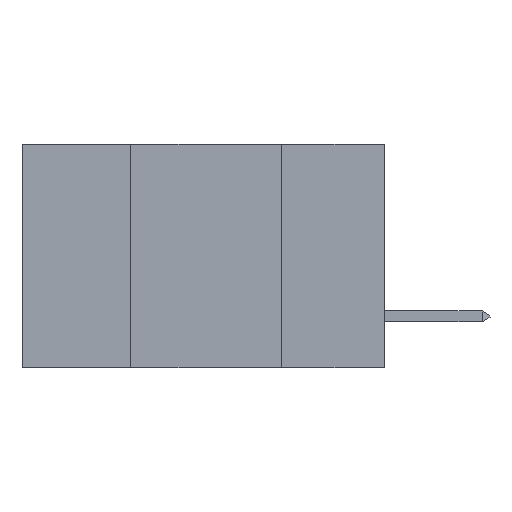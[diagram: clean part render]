
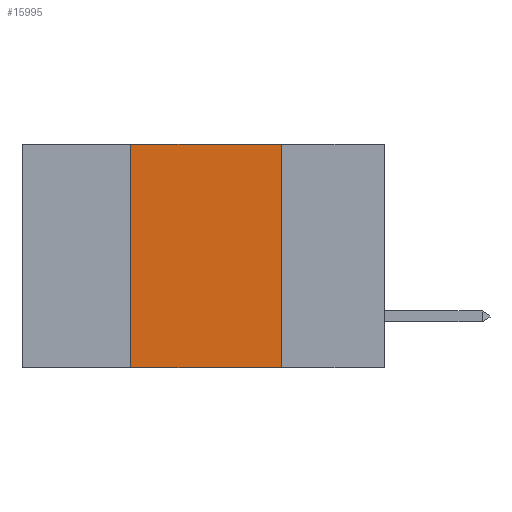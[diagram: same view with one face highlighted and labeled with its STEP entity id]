
A CAD part, left-side view. The second image highlights one B-rep face of the part: STEP entity #15995.
In plain terms, the highlighted planar face has unit normal (-1, 0, 0).
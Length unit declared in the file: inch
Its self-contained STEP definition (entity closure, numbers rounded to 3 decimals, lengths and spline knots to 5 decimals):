
#374 = EDGE_CURVE ( 'NONE', #13476, #15386, #3589, .T. ) ;
#1510 = CARTESIAN_POINT ( 'NONE',  ( 0., 0.42, -0.37 ) ) ;
#1744 = DIRECTION ( 'NONE',  ( 0., 0., 1. ) ) ;
#2388 = CARTESIAN_POINT ( 'NONE',  ( 0., 0.42, 0. ) ) ;
#2417 = EDGE_CURVE ( 'NONE', #13632, #15386, #13837, .T. ) ;
#2480 = DIRECTION ( 'NONE',  ( 0., -1., 0. ) ) ;
#3125 = VECTOR ( 'NONE', #2480, 39.37008 ) ;
#3589 = LINE ( 'NONE', #6136, #9292 ) ;
#3931 = CARTESIAN_POINT ( 'NONE',  ( 0., 0.6, 0. ) ) ;
#4759 = ORIENTED_EDGE ( 'NONE', *, *, #2417, .T. ) ;
#5179 = VECTOR ( 'NONE', #1744, 39.37008 ) ;
#5359 = ORIENTED_EDGE ( 'NONE', *, *, #374, .F. ) ;
#6024 = DIRECTION ( 'NONE',  ( 0., 0., -1. ) ) ;
#6128 = CARTESIAN_POINT ( 'NONE',  ( 0., 0.42, 0. ) ) ;
#6136 = CARTESIAN_POINT ( 'NONE',  ( 0., 0.17, 0. ) ) ;
#6312 = VERTEX_POINT ( 'NONE', #2388 ) ;
#6622 = DIRECTION ( 'NONE',  ( 0., -1., 0. ) ) ;
#7941 = LINE ( 'NONE', #13098, #18543 ) ;
#8242 = DIRECTION ( 'NONE',  ( 1., 0., 0. ) ) ;
#9292 = VECTOR ( 'NONE', #6024, 39.37008 ) ;
#10868 = LINE ( 'NONE', #6128, #5179 ) ;
#12105 = EDGE_CURVE ( 'NONE', #6312, #13476, #7941, .T. ) ;
#13098 = CARTESIAN_POINT ( 'NONE',  ( 0., 0.6, 0. ) ) ;
#13476 = VERTEX_POINT ( 'NONE', #17970 ) ;
#13632 = VERTEX_POINT ( 'NONE', #1510 ) ;
#13837 = LINE ( 'NONE', #17589, #3125 ) ;
#14036 = ORIENTED_EDGE ( 'NONE', *, *, #12105, .F. ) ;
#14387 = CARTESIAN_POINT ( 'NONE',  ( 0., 0.17, -0.37 ) ) ;
#15386 = VERTEX_POINT ( 'NONE', #14387 ) ;
#15995 = ADVANCED_FACE ( 'NONE', ( #18594 ), #24990, .F. ) ;
#16824 = EDGE_LOOP ( 'NONE', ( #5359, #14036, #22547, #4759 ) ) ;
#17589 = CARTESIAN_POINT ( 'NONE',  ( 0., 0.6, -0.37 ) ) ;
#17970 = CARTESIAN_POINT ( 'NONE',  ( 0., 0.17, 0. ) ) ;
#18028 = AXIS2_PLACEMENT_3D ( 'NONE', #3931, #8242, #22948 ) ;
#18543 = VECTOR ( 'NONE', #6622, 39.37008 ) ;
#18594 = FACE_OUTER_BOUND ( 'NONE', #16824, .T. ) ;
#19532 = EDGE_CURVE ( 'NONE', #13632, #6312, #10868, .T. ) ;
#22547 = ORIENTED_EDGE ( 'NONE', *, *, #19532, .F. ) ;
#22948 = DIRECTION ( 'NONE',  ( 0., 0., -1. ) ) ;
#24990 = PLANE ( 'NONE',  #18028 ) ;
